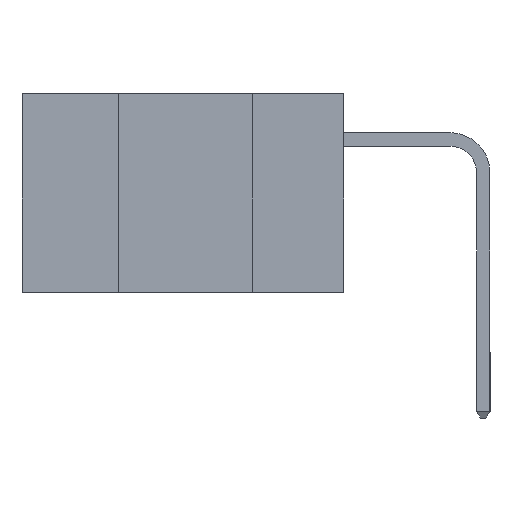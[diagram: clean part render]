
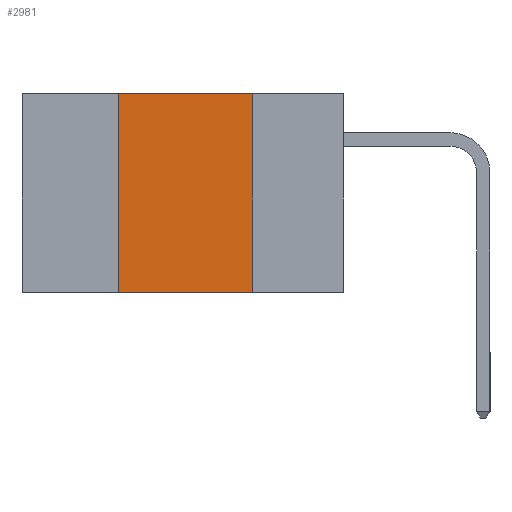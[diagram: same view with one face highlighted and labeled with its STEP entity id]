
A CAD part, left-side view. The second image highlights one B-rep face of the part: STEP entity #2981.
In plain terms, the highlighted planar face has unit normal (-1, 0, 0).
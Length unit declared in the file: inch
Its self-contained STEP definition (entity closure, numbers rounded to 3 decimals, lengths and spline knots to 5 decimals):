
#29 = VECTOR ( 'NONE', #5825, 39.37008 ) ;
#291 = AXIS2_PLACEMENT_3D ( 'NONE', #3922, #4989, #2093 ) ;
#292 = FACE_OUTER_BOUND ( 'NONE', #908, .T. ) ;
#293 = VECTOR ( 'NONE', #11332, 39.37008 ) ;
#908 = EDGE_LOOP ( 'NONE', ( #8760, #10664, #7602, #6273 ) ) ;
#1820 = LINE ( 'NONE', #11441, #293 ) ;
#2093 = DIRECTION ( 'NONE',  ( 0., 0., -1. ) ) ;
#2395 = LINE ( 'NONE', #11969, #2649 ) ;
#2463 = DIRECTION ( 'NONE',  ( 0., 0., 1. ) ) ;
#2551 = VERTEX_POINT ( 'NONE', #4476 ) ;
#2649 = VECTOR ( 'NONE', #2463, 39.37008 ) ;
#2981 = ADVANCED_FACE ( 'NONE', ( #292 ), #11655, .F. ) ;
#3190 = VECTOR ( 'NONE', #3749, 39.37008 ) ;
#3749 = DIRECTION ( 'NONE',  ( 0., -1., 0. ) ) ;
#3750 = EDGE_CURVE ( 'NONE', #2551, #4555, #6784, .T. ) ;
#3922 = CARTESIAN_POINT ( 'NONE',  ( 0., 0.6, 0. ) ) ;
#4092 = CARTESIAN_POINT ( 'NONE',  ( 0., 0.42, -0.37 ) ) ;
#4297 = VERTEX_POINT ( 'NONE', #12214 ) ;
#4432 = EDGE_CURVE ( 'NONE', #10172, #4555, #1820, .T. ) ;
#4476 = CARTESIAN_POINT ( 'NONE',  ( 0., 0.17, 0. ) ) ;
#4555 = VERTEX_POINT ( 'NONE', #7668 ) ;
#4655 = LINE ( 'NONE', #8546, #3190 ) ;
#4989 = DIRECTION ( 'NONE',  ( 1., 0., 0. ) ) ;
#5825 = DIRECTION ( 'NONE',  ( 0., 0., -1. ) ) ;
#6273 = ORIENTED_EDGE ( 'NONE', *, *, #4432, .T. ) ;
#6477 = EDGE_CURVE ( 'NONE', #4297, #2551, #4655, .T. ) ;
#6784 = LINE ( 'NONE', #8845, #29 ) ;
#7602 = ORIENTED_EDGE ( 'NONE', *, *, #9812, .F. ) ;
#7668 = CARTESIAN_POINT ( 'NONE',  ( 0., 0.17, -0.37 ) ) ;
#8546 = CARTESIAN_POINT ( 'NONE',  ( 0., 0.6, 0. ) ) ;
#8760 = ORIENTED_EDGE ( 'NONE', *, *, #3750, .F. ) ;
#8845 = CARTESIAN_POINT ( 'NONE',  ( 0., 0.17, -0.37 ) ) ;
#9812 = EDGE_CURVE ( 'NONE', #10172, #4297, #2395, .T. ) ;
#10172 = VERTEX_POINT ( 'NONE', #4092 ) ;
#10664 = ORIENTED_EDGE ( 'NONE', *, *, #6477, .F. ) ;
#11332 = DIRECTION ( 'NONE',  ( 0., -1., 0. ) ) ;
#11441 = CARTESIAN_POINT ( 'NONE',  ( 0., 0.6, -0.37 ) ) ;
#11655 = PLANE ( 'NONE',  #291 ) ;
#11969 = CARTESIAN_POINT ( 'NONE',  ( 0., 0.42, -0.37 ) ) ;
#12214 = CARTESIAN_POINT ( 'NONE',  ( 0., 0.42, 0. ) ) ;
